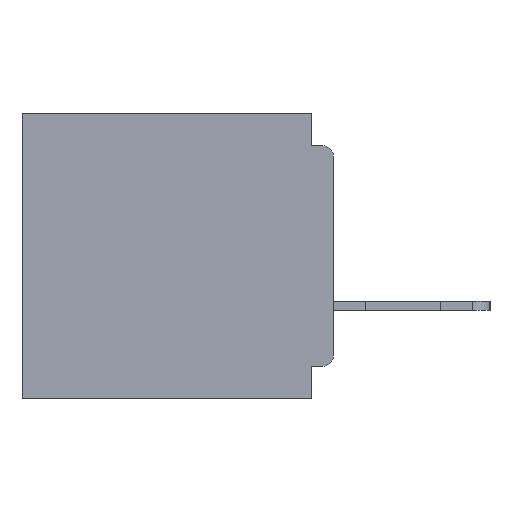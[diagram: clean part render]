
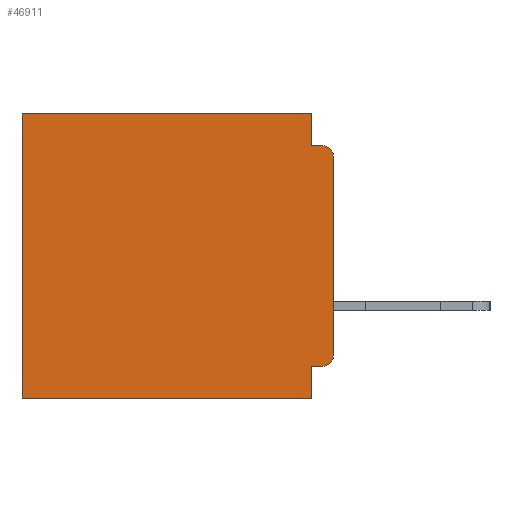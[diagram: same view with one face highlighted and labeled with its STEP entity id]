
A CAD part, left-side view. The second image highlights one B-rep face of the part: STEP entity #46911.
In plain terms, the highlighted planar face has unit normal (-1, 0, 0).
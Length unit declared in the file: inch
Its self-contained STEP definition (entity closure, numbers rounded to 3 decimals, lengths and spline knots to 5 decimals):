
#172 = CARTESIAN_POINT ( 'NONE',  ( 0.3, 0., -0.355 ) ) ;
#1356 = CARTESIAN_POINT ( 'NONE',  ( 0.3, 0., 0. ) ) ;
#1442 = ORIENTED_EDGE ( 'NONE', *, *, #14842, .T. ) ;
#3990 = VECTOR ( 'NONE', #49622, 39.37008 ) ;
#4284 = EDGE_CURVE ( 'NONE', #41540, #17514, #7643, .T. ) ;
#4390 = EDGE_CURVE ( 'NONE', #24585, #7484, #35328, .T. ) ;
#4956 = LINE ( 'NONE', #172, #46075 ) ;
#5023 = LINE ( 'NONE', #20454, #14791 ) ;
#5319 = LINE ( 'NONE', #45488, #3990 ) ;
#5364 = EDGE_CURVE ( 'NONE', #41540, #49859, #26754, .T. ) ;
#7484 = VERTEX_POINT ( 'NONE', #32645 ) ;
#7643 = LINE ( 'NONE', #47959, #17384 ) ;
#12529 = VERTEX_POINT ( 'NONE', #24860 ) ;
#13113 = CIRCLE ( 'NONE', #28011, 0.015 ) ;
#14789 = VERTEX_POINT ( 'NONE', #36670 ) ;
#14791 = VECTOR ( 'NONE', #36854, 39.37008 ) ;
#14842 = EDGE_CURVE ( 'NONE', #18300, #7484, #13113, .T. ) ;
#15410 = CARTESIAN_POINT ( 'NONE',  ( 0.3, 0.031, -0.4 ) ) ;
#15594 = CARTESIAN_POINT ( 'NONE',  ( 0.3, 0., -0.045 ) ) ;
#15941 = CARTESIAN_POINT ( 'NONE',  ( 0.3, 0., -0.4 ) ) ;
#17384 = VECTOR ( 'NONE', #48141, 39.37008 ) ;
#17514 = VERTEX_POINT ( 'NONE', #31496 ) ;
#18197 = CARTESIAN_POINT ( 'NONE',  ( 0.3, 0.015, -0.06 ) ) ;
#18300 = VERTEX_POINT ( 'NONE', #49037 ) ;
#19247 = FACE_OUTER_BOUND ( 'NONE', #28513, .T. ) ;
#20454 = CARTESIAN_POINT ( 'NONE',  ( 0.3, 0., -0.4 ) ) ;
#20769 = CARTESIAN_POINT ( 'NONE',  ( 0.3, 0.015, -0.34 ) ) ;
#21337 = ORIENTED_EDGE ( 'NONE', *, *, #4284, .F. ) ;
#22135 = DIRECTION ( 'NONE',  ( 0., 1., 0. ) ) ;
#22331 = DIRECTION ( 'NONE',  ( 0., 0., -1. ) ) ;
#23572 = VERTEX_POINT ( 'NONE', #25702 ) ;
#23839 = DIRECTION ( 'NONE',  ( 0., 0., -1. ) ) ;
#24041 = DIRECTION ( 'NONE',  ( 0., -1., 0. ) ) ;
#24403 = LINE ( 'NONE', #15594, #44825 ) ;
#24585 = VERTEX_POINT ( 'NONE', #36838 ) ;
#24860 = CARTESIAN_POINT ( 'NONE',  ( 0.3, 0.031, -0.355 ) ) ;
#24863 = DIRECTION ( 'NONE',  ( 0., 0., -1. ) ) ;
#24907 = DIRECTION ( 'NONE',  ( 0., 0., -1. ) ) ;
#25702 = CARTESIAN_POINT ( 'NONE',  ( 0.3, 0.015, -0.045 ) ) ;
#26754 = LINE ( 'NONE', #1356, #37580 ) ;
#27893 = ORIENTED_EDGE ( 'NONE', *, *, #4390, .F. ) ;
#28011 = AXIS2_PLACEMENT_3D ( 'NONE', #20769, #49304, #24863 ) ;
#28361 = DIRECTION ( 'NONE',  ( 0., 0., -1. ) ) ;
#28513 = EDGE_LOOP ( 'NONE', ( #27893, #49054, #49259, #21337, #34470, #46952, #30213, #50554, #40805, #1442 ) ) ;
#29273 = EDGE_CURVE ( 'NONE', #46445, #14789, #5023, .T. ) ;
#30213 = ORIENTED_EDGE ( 'NONE', *, *, #29273, .F. ) ;
#30385 = EDGE_CURVE ( 'NONE', #17514, #23572, #24403, .T. ) ;
#31398 = EDGE_CURVE ( 'NONE', #24585, #23572, #35825, .T. ) ;
#31481 = LINE ( 'NONE', #49349, #53124 ) ;
#31496 = CARTESIAN_POINT ( 'NONE',  ( 0.3, 0.031, -0.045 ) ) ;
#31914 = PLANE ( 'NONE',  #53366 ) ;
#32645 = CARTESIAN_POINT ( 'NONE',  ( 0.3, 0., -0.34 ) ) ;
#33094 = EDGE_CURVE ( 'NONE', #49859, #14789, #5319, .T. ) ;
#33506 = DIRECTION ( 'NONE',  ( 0., 1., 0. ) ) ;
#34470 = ORIENTED_EDGE ( 'NONE', *, *, #5364, .T. ) ;
#35328 = LINE ( 'NONE', #15941, #44847 ) ;
#35825 = CIRCLE ( 'NONE', #44624, 0.015 ) ;
#36013 = CARTESIAN_POINT ( 'NONE',  ( 0.3, 0., -0.4 ) ) ;
#36670 = CARTESIAN_POINT ( 'NONE',  ( 0.3, 0.437, -0.4 ) ) ;
#36838 = CARTESIAN_POINT ( 'NONE',  ( 0.3, 0., -0.06 ) ) ;
#36854 = DIRECTION ( 'NONE',  ( 0., 1., 0. ) ) ;
#37580 = VECTOR ( 'NONE', #22135, 39.37008 ) ;
#39555 = EDGE_CURVE ( 'NONE', #18300, #12529, #4956, .T. ) ;
#40016 = CARTESIAN_POINT ( 'NONE',  ( 0.3, 0.437, 0. ) ) ;
#40805 = ORIENTED_EDGE ( 'NONE', *, *, #39555, .F. ) ;
#41540 = VERTEX_POINT ( 'NONE', #50233 ) ;
#43887 = EDGE_CURVE ( 'NONE', #12529, #46445, #31481, .T. ) ;
#44624 = AXIS2_PLACEMENT_3D ( 'NONE', #18197, #46746, #22331 ) ;
#44825 = VECTOR ( 'NONE', #24041, 39.37008 ) ;
#44847 = VECTOR ( 'NONE', #28361, 39.37008 ) ;
#45488 = CARTESIAN_POINT ( 'NONE',  ( 0.3, 0.437, -0.4 ) ) ;
#46075 = VECTOR ( 'NONE', #33506, 39.37008 ) ;
#46445 = VERTEX_POINT ( 'NONE', #15410 ) ;
#46746 = DIRECTION ( 'NONE',  ( -1., 0., 0. ) ) ;
#46911 = ADVANCED_FACE ( 'NONE', ( #19247 ), #31914, .F. ) ;
#46952 = ORIENTED_EDGE ( 'NONE', *, *, #33094, .T. ) ;
#47959 = CARTESIAN_POINT ( 'NONE',  ( 0.3, 0.031, 0. ) ) ;
#48141 = DIRECTION ( 'NONE',  ( 0., 0., -1. ) ) ;
#48274 = DIRECTION ( 'NONE',  ( 1., 0., 0. ) ) ;
#49037 = CARTESIAN_POINT ( 'NONE',  ( 0.3, 0.015, -0.355 ) ) ;
#49054 = ORIENTED_EDGE ( 'NONE', *, *, #31398, .T. ) ;
#49259 = ORIENTED_EDGE ( 'NONE', *, *, #30385, .F. ) ;
#49304 = DIRECTION ( 'NONE',  ( -1., 0., 0. ) ) ;
#49349 = CARTESIAN_POINT ( 'NONE',  ( 0.3, 0.031, -0.4 ) ) ;
#49622 = DIRECTION ( 'NONE',  ( 0., 0., -1. ) ) ;
#49859 = VERTEX_POINT ( 'NONE', #40016 ) ;
#50233 = CARTESIAN_POINT ( 'NONE',  ( 0.3, 0.031, 0. ) ) ;
#50554 = ORIENTED_EDGE ( 'NONE', *, *, #43887, .F. ) ;
#53124 = VECTOR ( 'NONE', #24907, 39.37008 ) ;
#53366 = AXIS2_PLACEMENT_3D ( 'NONE', #36013, #48274, #23839 ) ;
